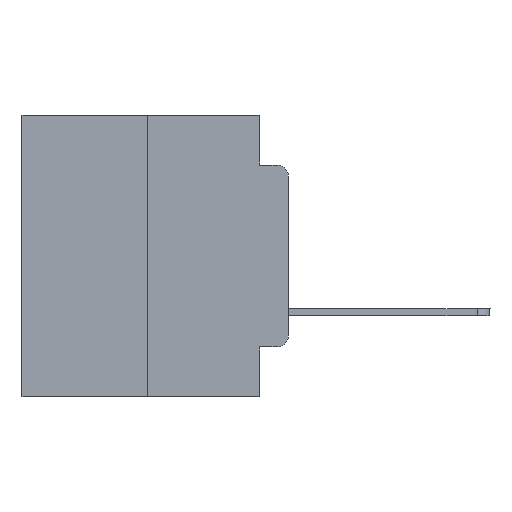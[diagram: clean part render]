
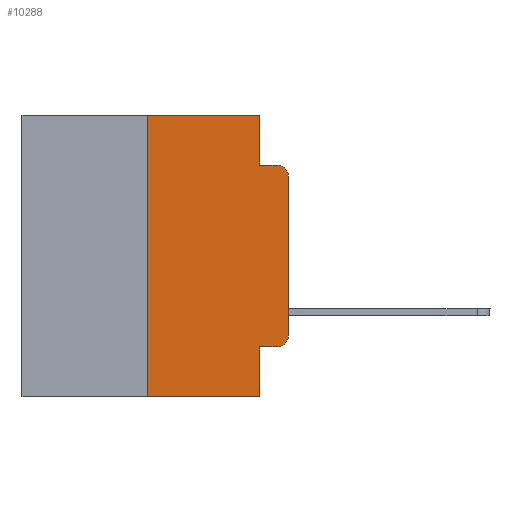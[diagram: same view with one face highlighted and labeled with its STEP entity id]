
A CAD part, left-side view. The second image highlights one B-rep face of the part: STEP entity #10288.
In plain terms, the highlighted planar face has unit normal (-1, 0, 0).
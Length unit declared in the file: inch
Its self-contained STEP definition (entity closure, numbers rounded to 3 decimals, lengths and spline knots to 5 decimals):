
#283 = ORIENTED_EDGE ( 'NONE', *, *, #1101, .F. ) ;
#732 = CARTESIAN_POINT ( 'NONE',  ( 0., 0.02, -0.4115 ) ) ;
#934 = AXIS2_PLACEMENT_3D ( 'NONE', #10366, #14437, #14057 ) ;
#1094 = EDGE_CURVE ( 'NONE', #16140, #9052, #1507, .T. ) ;
#1101 = EDGE_CURVE ( 'NONE', #9052, #1853, #14410, .T. ) ;
#1193 = EDGE_LOOP ( 'NONE', ( #23658, #2163, #10283, #283, #18463, #24559, #13512, #8445, #16796, #21799 ) ) ;
#1203 = CARTESIAN_POINT ( 'NONE',  ( 0., 0., -0.3915 ) ) ;
#1414 = DIRECTION ( 'NONE',  ( 0., -1., 0. ) ) ;
#1507 = LINE ( 'NONE', #19987, #17250 ) ;
#1830 = CARTESIAN_POINT ( 'NONE',  ( 0., 0.051, -0.0885 ) ) ;
#1853 = VERTEX_POINT ( 'NONE', #1830 ) ;
#2163 = ORIENTED_EDGE ( 'NONE', *, *, #10343, .T. ) ;
#2478 = CARTESIAN_POINT ( 'NONE',  ( 0., 0.25, 0. ) ) ;
#3006 = LINE ( 'NONE', #2478, #13432 ) ;
#3051 = DIRECTION ( 'NONE',  ( -1., 0., 0. ) ) ;
#3914 = CARTESIAN_POINT ( 'NONE',  ( 0., 0.051, 0. ) ) ;
#4321 = EDGE_CURVE ( 'NONE', #6930, #9348, #17017, .T. ) ;
#6838 = DIRECTION ( 'NONE',  ( 0., 0., 1. ) ) ;
#6930 = VERTEX_POINT ( 'NONE', #1203 ) ;
#6988 = DIRECTION ( 'NONE',  ( 0., 0., 1. ) ) ;
#7225 = VERTEX_POINT ( 'NONE', #12394 ) ;
#7860 = CARTESIAN_POINT ( 'NONE',  ( 0., 0.02, -0.0885 ) ) ;
#8101 = DIRECTION ( 'NONE',  ( 0., 0., -1. ) ) ;
#8111 = VECTOR ( 'NONE', #19479, 39.37008 ) ;
#8445 = ORIENTED_EDGE ( 'NONE', *, *, #23516, .F. ) ;
#9052 = VERTEX_POINT ( 'NONE', #14640 ) ;
#9330 = CARTESIAN_POINT ( 'NONE',  ( 0., 0.051, -0.4115 ) ) ;
#9334 = LINE ( 'NONE', #21751, #26063 ) ;
#9348 = VERTEX_POINT ( 'NONE', #14098 ) ;
#10074 = CARTESIAN_POINT ( 'NONE',  ( 0., 0.473, 0. ) ) ;
#10283 = ORIENTED_EDGE ( 'NONE', *, *, #25807, .F. ) ;
#10288 = ADVANCED_FACE ( 'NONE', ( #19994 ), #14158, .F. ) ;
#10343 = EDGE_CURVE ( 'NONE', #9348, #25790, #23257, .T. ) ;
#10366 = CARTESIAN_POINT ( 'NONE',  ( 0., 0.02, -0.3915 ) ) ;
#10909 = VECTOR ( 'NONE', #20380, 39.37008 ) ;
#11150 = VECTOR ( 'NONE', #22380, 39.37008 ) ;
#11918 = DIRECTION ( 'NONE',  ( 0., -1., 0. ) ) ;
#12394 = CARTESIAN_POINT ( 'NONE',  ( 0., 0.25, -0.5 ) ) ;
#13061 = CARTESIAN_POINT ( 'NONE',  ( 0., 0.02, -0.1085 ) ) ;
#13369 = CARTESIAN_POINT ( 'NONE',  ( 0., 0.25, 0. ) ) ;
#13399 = LINE ( 'NONE', #3914, #8111 ) ;
#13432 = VECTOR ( 'NONE', #6838, 39.37008 ) ;
#13512 = ORIENTED_EDGE ( 'NONE', *, *, #14150, .T. ) ;
#14057 = DIRECTION ( 'NONE',  ( 0., 0., -1. ) ) ;
#14098 = CARTESIAN_POINT ( 'NONE',  ( 0., 0., -0.1085 ) ) ;
#14150 = EDGE_CURVE ( 'NONE', #7225, #25170, #18256, .T. ) ;
#14158 = PLANE ( 'NONE',  #14393 ) ;
#14160 = CARTESIAN_POINT ( 'NONE',  ( 0., 0.473, -0.5 ) ) ;
#14393 = AXIS2_PLACEMENT_3D ( 'NONE', #10074, #18125, #8101 ) ;
#14410 = LINE ( 'NONE', #18635, #10909 ) ;
#14437 = DIRECTION ( 'NONE',  ( -1., 0., 0. ) ) ;
#14640 = CARTESIAN_POINT ( 'NONE',  ( 0., 0.051, 0. ) ) ;
#15229 = AXIS2_PLACEMENT_3D ( 'NONE', #13061, #3051, #24473 ) ;
#15822 = CARTESIAN_POINT ( 'NONE',  ( 0., 0.051, -0.5 ) ) ;
#16140 = VERTEX_POINT ( 'NONE', #13369 ) ;
#16796 = ORIENTED_EDGE ( 'NONE', *, *, #18766, .T. ) ;
#17017 = LINE ( 'NONE', #21109, #21434 ) ;
#17250 = VECTOR ( 'NONE', #11918, 39.37008 ) ;
#17410 = EDGE_CURVE ( 'NONE', #7225, #16140, #3006, .T. ) ;
#17559 = VERTEX_POINT ( 'NONE', #9330 ) ;
#18125 = DIRECTION ( 'NONE',  ( 1., 0., 0. ) ) ;
#18219 = CIRCLE ( 'NONE', #934, 0.02 ) ;
#18256 = LINE ( 'NONE', #14160, #21691 ) ;
#18463 = ORIENTED_EDGE ( 'NONE', *, *, #1094, .F. ) ;
#18635 = CARTESIAN_POINT ( 'NONE',  ( 0., 0.051, 0. ) ) ;
#18766 = EDGE_CURVE ( 'NONE', #17559, #25575, #9334, .T. ) ;
#19479 = DIRECTION ( 'NONE',  ( 0., 0., -1. ) ) ;
#19987 = CARTESIAN_POINT ( 'NONE',  ( 0., 0.473, 0. ) ) ;
#19994 = FACE_OUTER_BOUND ( 'NONE', #1193, .T. ) ;
#20380 = DIRECTION ( 'NONE',  ( 0., 0., -1. ) ) ;
#21109 = CARTESIAN_POINT ( 'NONE',  ( 0., 0., 0. ) ) ;
#21434 = VECTOR ( 'NONE', #6988, 39.37008 ) ;
#21691 = VECTOR ( 'NONE', #22233, 39.37008 ) ;
#21751 = CARTESIAN_POINT ( 'NONE',  ( 0., 0.051, -0.4115 ) ) ;
#21799 = ORIENTED_EDGE ( 'NONE', *, *, #22390, .T. ) ;
#21989 = LINE ( 'NONE', #24236, #11150 ) ;
#22233 = DIRECTION ( 'NONE',  ( 0., -1., 0. ) ) ;
#22380 = DIRECTION ( 'NONE',  ( 0., -1., 0. ) ) ;
#22390 = EDGE_CURVE ( 'NONE', #25575, #6930, #18219, .T. ) ;
#23257 = CIRCLE ( 'NONE', #15229, 0.02 ) ;
#23516 = EDGE_CURVE ( 'NONE', #17559, #25170, #13399, .T. ) ;
#23658 = ORIENTED_EDGE ( 'NONE', *, *, #4321, .T. ) ;
#24236 = CARTESIAN_POINT ( 'NONE',  ( 0., 0.051, -0.0885 ) ) ;
#24473 = DIRECTION ( 'NONE',  ( 0., 0., -1. ) ) ;
#24559 = ORIENTED_EDGE ( 'NONE', *, *, #17410, .F. ) ;
#25170 = VERTEX_POINT ( 'NONE', #15822 ) ;
#25575 = VERTEX_POINT ( 'NONE', #732 ) ;
#25790 = VERTEX_POINT ( 'NONE', #7860 ) ;
#25807 = EDGE_CURVE ( 'NONE', #1853, #25790, #21989, .T. ) ;
#26063 = VECTOR ( 'NONE', #1414, 39.37008 ) ;
